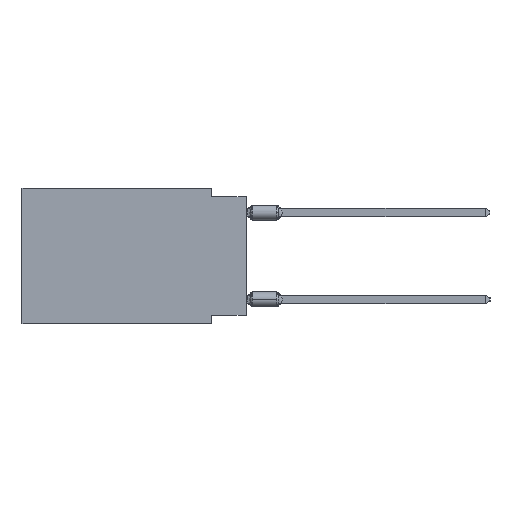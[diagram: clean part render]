
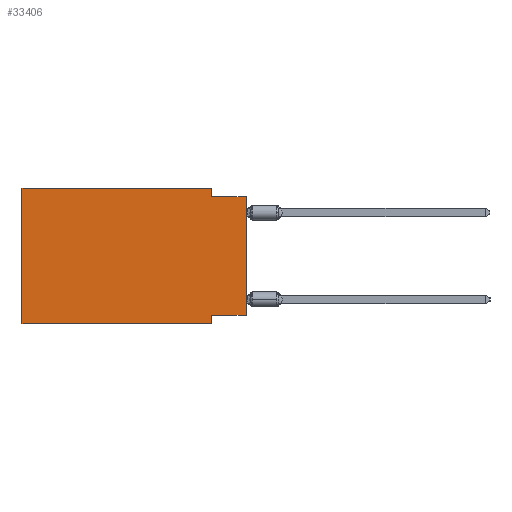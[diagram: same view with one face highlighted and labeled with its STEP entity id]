
A CAD part, left-side view. The second image highlights one B-rep face of the part: STEP entity #33406.
In plain terms, the highlighted planar face has unit normal (-1, 0, 0).
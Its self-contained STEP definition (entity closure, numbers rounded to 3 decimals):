
#362 = CARTESIAN_POINT ( 'NONE',  ( 0., 2.54, 0. ) ) ;
#785 = LINE ( 'NONE', #18705, #37825 ) ;
#967 = CARTESIAN_POINT ( 'NONE',  ( 0., 0., 0. ) ) ;
#984 = VECTOR ( 'NONE', #16754, 1000. ) ;
#2542 = CARTESIAN_POINT ( 'NONE',  ( 0., 16.383, -9.906 ) ) ;
#2867 = PLANE ( 'NONE',  #14484 ) ;
#3994 = LINE ( 'NONE', #40049, #44737 ) ;
#4576 = DIRECTION ( 'NONE',  ( 0., 0., -1. ) ) ;
#9267 = VECTOR ( 'NONE', #15345, 1000. ) ;
#9384 = LINE ( 'NONE', #2542, #16862 ) ;
#9694 = LINE ( 'NONE', #17228, #984 ) ;
#10058 = ORIENTED_EDGE ( 'NONE', *, *, #35233, .T. ) ;
#11340 = LINE ( 'NONE', #967, #9267 ) ;
#11563 = VECTOR ( 'NONE', #44501, 1000. ) ;
#14143 = CARTESIAN_POINT ( 'NONE',  ( 0., 2.54, -9.906 ) ) ;
#14484 = AXIS2_PLACEMENT_3D ( 'NONE', #38217, #24056, #16760 ) ;
#15345 = DIRECTION ( 'NONE',  ( 0., 0., 1. ) ) ;
#15456 = CARTESIAN_POINT ( 'NONE',  ( 0., 0., -9.271 ) ) ;
#15818 = CARTESIAN_POINT ( 'NONE',  ( 0., 2.54, -9.271 ) ) ;
#16754 = DIRECTION ( 'NONE',  ( 0., 1., 0. ) ) ;
#16760 = DIRECTION ( 'NONE',  ( 0., 0., -1. ) ) ;
#16862 = VECTOR ( 'NONE', #27742, 1000. ) ;
#17228 = CARTESIAN_POINT ( 'NONE',  ( 0., 0., -9.271 ) ) ;
#17529 = ORIENTED_EDGE ( 'NONE', *, *, #35150, .F. ) ;
#17599 = EDGE_CURVE ( 'NONE', #30597, #28867, #9694, .T. ) ;
#17902 = LINE ( 'NONE', #14143, #31091 ) ;
#18661 = ORIENTED_EDGE ( 'NONE', *, *, #24749, .F. ) ;
#18705 = CARTESIAN_POINT ( 'NONE',  ( 0., 16.383, 0. ) ) ;
#18829 = VERTEX_POINT ( 'NONE', #19394 ) ;
#19056 = DIRECTION ( 'NONE',  ( 0., -1., 0. ) ) ;
#19187 = ORIENTED_EDGE ( 'NONE', *, *, #41485, .F. ) ;
#19394 = CARTESIAN_POINT ( 'NONE',  ( 0., 0., -0.635 ) ) ;
#20853 = ORIENTED_EDGE ( 'NONE', *, *, #32966, .F. ) ;
#22355 = CARTESIAN_POINT ( 'NONE',  ( 0., 16.383, 0. ) ) ;
#22811 = CARTESIAN_POINT ( 'NONE',  ( 0., 2.54, -0.635 ) ) ;
#24056 = DIRECTION ( 'NONE',  ( 1., 0., 0. ) ) ;
#24749 = EDGE_CURVE ( 'NONE', #36518, #26865, #785, .T. ) ;
#25491 = VERTEX_POINT ( 'NONE', #43064 ) ;
#26460 = DIRECTION ( 'NONE',  ( 0., -1., 0. ) ) ;
#26865 = VERTEX_POINT ( 'NONE', #27468 ) ;
#27468 = CARTESIAN_POINT ( 'NONE',  ( 0., 2.54, 0. ) ) ;
#27742 = DIRECTION ( 'NONE',  ( 0., -1., 0. ) ) ;
#28508 = DIRECTION ( 'NONE',  ( 0., 0., -1. ) ) ;
#28867 = VERTEX_POINT ( 'NONE', #15818 ) ;
#30597 = VERTEX_POINT ( 'NONE', #15456 ) ;
#31091 = VECTOR ( 'NONE', #28508, 1000. ) ;
#32654 = EDGE_CURVE ( 'NONE', #30597, #18829, #11340, .T. ) ;
#32966 = EDGE_CURVE ( 'NONE', #28867, #46427, #17902, .T. ) ;
#33334 = LINE ( 'NONE', #362, #34132 ) ;
#33340 = ORIENTED_EDGE ( 'NONE', *, *, #35124, .F. ) ;
#33406 = ADVANCED_FACE ( 'NONE', ( #35145 ), #2867, .F. ) ;
#34132 = VECTOR ( 'NONE', #4576, 1000. ) ;
#34813 = CARTESIAN_POINT ( 'NONE',  ( 0., 16.383, 0. ) ) ;
#35124 = EDGE_CURVE ( 'NONE', #25491, #36518, #36949, .T. ) ;
#35145 = FACE_OUTER_BOUND ( 'NONE', #40972, .T. ) ;
#35150 = EDGE_CURVE ( 'NONE', #35177, #18829, #3994, .T. ) ;
#35177 = VERTEX_POINT ( 'NONE', #22811 ) ;
#35233 = EDGE_CURVE ( 'NONE', #25491, #46427, #9384, .T. ) ;
#36055 = ORIENTED_EDGE ( 'NONE', *, *, #17599, .F. ) ;
#36518 = VERTEX_POINT ( 'NONE', #34813 ) ;
#36949 = LINE ( 'NONE', #22355, #11563 ) ;
#37825 = VECTOR ( 'NONE', #26460, 1000. ) ;
#38217 = CARTESIAN_POINT ( 'NONE',  ( 0., 16.383, 0. ) ) ;
#40049 = CARTESIAN_POINT ( 'NONE',  ( 0., 0., -0.635 ) ) ;
#40948 = CARTESIAN_POINT ( 'NONE',  ( 0., 2.54, -9.906 ) ) ;
#40972 = EDGE_LOOP ( 'NONE', ( #44299, #17529, #19187, #18661, #33340, #10058, #20853, #36055 ) ) ;
#41485 = EDGE_CURVE ( 'NONE', #26865, #35177, #33334, .T. ) ;
#43064 = CARTESIAN_POINT ( 'NONE',  ( 0., 16.383, -9.906 ) ) ;
#44299 = ORIENTED_EDGE ( 'NONE', *, *, #32654, .T. ) ;
#44501 = DIRECTION ( 'NONE',  ( 0., 0., 1. ) ) ;
#44737 = VECTOR ( 'NONE', #19056, 1000. ) ;
#46427 = VERTEX_POINT ( 'NONE', #40948 ) ;
